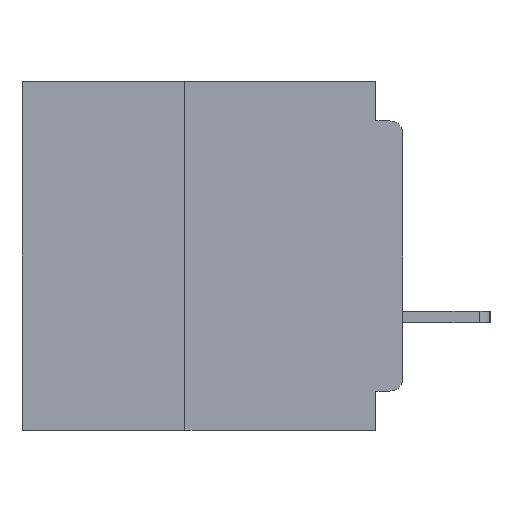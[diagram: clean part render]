
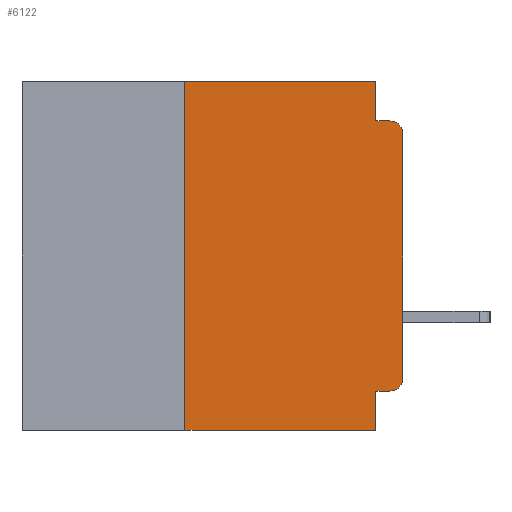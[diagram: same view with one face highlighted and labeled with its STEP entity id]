
A CAD part, left-side view. The second image highlights one B-rep face of the part: STEP entity #6122.
In plain terms, the highlighted planar face has unit normal (-1, 0, 0).
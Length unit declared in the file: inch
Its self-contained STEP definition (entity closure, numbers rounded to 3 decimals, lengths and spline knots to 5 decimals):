
#371 = ORIENTED_EDGE ( 'NONE', *, *, #23966, .T. ) ;
#382 = CARTESIAN_POINT ( 'NONE',  ( 0., 0.25, -0.4 ) ) ;
#475 = CIRCLE ( 'NONE', #38629, 0.015 ) ;
#1666 = VERTEX_POINT ( 'NONE', #8540 ) ;
#4003 = VERTEX_POINT ( 'NONE', #382 ) ;
#4031 = ORIENTED_EDGE ( 'NONE', *, *, #8198, .T. ) ;
#5573 = EDGE_CURVE ( 'NONE', #4003, #1666, #17565, .T. ) ;
#6122 = ADVANCED_FACE ( 'NONE', ( #43134 ), #41842, .F. ) ;
#7147 = CARTESIAN_POINT ( 'NONE',  ( 0., 0.015, -0.355 ) ) ;
#7319 = LINE ( 'NONE', #8482, #46742 ) ;
#7358 = VECTOR ( 'NONE', #42615, 39.37008 ) ;
#8198 = EDGE_CURVE ( 'NONE', #46707, #48323, #47639, .T. ) ;
#8482 = CARTESIAN_POINT ( 'NONE',  ( 0., 0.437, 0. ) ) ;
#8540 = CARTESIAN_POINT ( 'NONE',  ( 0., 0.031, -0.4 ) ) ;
#10639 = VECTOR ( 'NONE', #27097, 39.37008 ) ;
#11335 = LINE ( 'NONE', #21030, #31790 ) ;
#12871 = VERTEX_POINT ( 'NONE', #7147 ) ;
#12902 = AXIS2_PLACEMENT_3D ( 'NONE', #16876, #43560, #20738 ) ;
#13273 = CARTESIAN_POINT ( 'NONE',  ( 0., 0.437, -0.4 ) ) ;
#13705 = DIRECTION ( 'NONE',  ( 0., -1., 0. ) ) ;
#13744 = DIRECTION ( 'NONE',  ( 0., 0., 1. ) ) ;
#15393 = ORIENTED_EDGE ( 'NONE', *, *, #5573, .T. ) ;
#15849 = VERTEX_POINT ( 'NONE', #41831 ) ;
#16168 = EDGE_CURVE ( 'NONE', #4003, #17813, #24903, .T. ) ;
#16334 = DIRECTION ( 'NONE',  ( -1., 0., 0. ) ) ;
#16491 = CARTESIAN_POINT ( 'NONE',  ( 0., 0., -0.355 ) ) ;
#16876 = CARTESIAN_POINT ( 'NONE',  ( 0., 0.015, -0.06 ) ) ;
#16954 = EDGE_CURVE ( 'NONE', #17813, #47381, #7319, .T. ) ;
#17565 = LINE ( 'NONE', #13273, #18763 ) ;
#17813 = VERTEX_POINT ( 'NONE', #36691 ) ;
#17838 = ORIENTED_EDGE ( 'NONE', *, *, #25099, .F. ) ;
#18763 = VECTOR ( 'NONE', #13705, 39.37008 ) ;
#19045 = ORIENTED_EDGE ( 'NONE', *, *, #48656, .F. ) ;
#19424 = VECTOR ( 'NONE', #13744, 39.37008 ) ;
#19915 = LINE ( 'NONE', #16491, #27682 ) ;
#20049 = EDGE_LOOP ( 'NONE', ( #371, #4031, #19045, #44079, #21466, #37556, #15393, #22036, #17838, #45035 ) ) ;
#20738 = DIRECTION ( 'NONE',  ( 0., 0., -1. ) ) ;
#21030 = CARTESIAN_POINT ( 'NONE',  ( 0., 0., -0.045 ) ) ;
#21466 = ORIENTED_EDGE ( 'NONE', *, *, #16954, .F. ) ;
#22036 = ORIENTED_EDGE ( 'NONE', *, *, #36797, .F. ) ;
#22149 = LINE ( 'NONE', #38689, #10639 ) ;
#23005 = VERTEX_POINT ( 'NONE', #30158 ) ;
#23358 = CARTESIAN_POINT ( 'NONE',  ( 0., 0.031, -0.045 ) ) ;
#23966 = EDGE_CURVE ( 'NONE', #15849, #46707, #39679, .T. ) ;
#24005 = DIRECTION ( 'NONE',  ( 0., -1., 0. ) ) ;
#24903 = LINE ( 'NONE', #38187, #26095 ) ;
#25099 = EDGE_CURVE ( 'NONE', #12871, #23005, #19915, .T. ) ;
#25739 = CARTESIAN_POINT ( 'NONE',  ( 0., 0.015, -0.045 ) ) ;
#26095 = VECTOR ( 'NONE', #30747, 39.37008 ) ;
#26703 = EDGE_CURVE ( 'NONE', #47381, #49003, #22149, .T. ) ;
#26773 = EDGE_CURVE ( 'NONE', #12871, #15849, #475, .T. ) ;
#27097 = DIRECTION ( 'NONE',  ( 0., 0., -1. ) ) ;
#27682 = VECTOR ( 'NONE', #43173, 39.37008 ) ;
#30158 = CARTESIAN_POINT ( 'NONE',  ( 0., 0.031, -0.355 ) ) ;
#30747 = DIRECTION ( 'NONE',  ( 0., 0., 1. ) ) ;
#31790 = VECTOR ( 'NONE', #40145, 39.37008 ) ;
#36666 = CARTESIAN_POINT ( 'NONE',  ( 0., 0., 0. ) ) ;
#36691 = CARTESIAN_POINT ( 'NONE',  ( 0., 0.25, 0. ) ) ;
#36797 = EDGE_CURVE ( 'NONE', #23005, #1666, #49130, .T. ) ;
#37556 = ORIENTED_EDGE ( 'NONE', *, *, #16168, .F. ) ;
#38187 = CARTESIAN_POINT ( 'NONE',  ( 0., 0.25, -0.4 ) ) ;
#38629 = AXIS2_PLACEMENT_3D ( 'NONE', #39178, #16334, #43012 ) ;
#38689 = CARTESIAN_POINT ( 'NONE',  ( 0., 0.031, 0. ) ) ;
#38771 = CARTESIAN_POINT ( 'NONE',  ( 0., 0.031, -0.4 ) ) ;
#39178 = CARTESIAN_POINT ( 'NONE',  ( 0., 0.015, -0.34 ) ) ;
#39679 = LINE ( 'NONE', #36666, #19424 ) ;
#39924 = CARTESIAN_POINT ( 'NONE',  ( 0., 0., -0.06 ) ) ;
#40145 = DIRECTION ( 'NONE',  ( 0., -1., 0. ) ) ;
#41303 = DIRECTION ( 'NONE',  ( 0., 0., -1. ) ) ;
#41416 = DIRECTION ( 'NONE',  ( 1., 0., 0. ) ) ;
#41688 = CARTESIAN_POINT ( 'NONE',  ( 0., 0.437, 0. ) ) ;
#41831 = CARTESIAN_POINT ( 'NONE',  ( 0., 0., -0.34 ) ) ;
#41842 = PLANE ( 'NONE',  #48625 ) ;
#42615 = DIRECTION ( 'NONE',  ( 0., 0., -1. ) ) ;
#42915 = CARTESIAN_POINT ( 'NONE',  ( 0., 0.031, 0. ) ) ;
#43012 = DIRECTION ( 'NONE',  ( 0., 0., -1. ) ) ;
#43134 = FACE_OUTER_BOUND ( 'NONE', #20049, .T. ) ;
#43173 = DIRECTION ( 'NONE',  ( 0., 1., 0. ) ) ;
#43560 = DIRECTION ( 'NONE',  ( -1., 0., 0. ) ) ;
#44079 = ORIENTED_EDGE ( 'NONE', *, *, #26703, .F. ) ;
#45035 = ORIENTED_EDGE ( 'NONE', *, *, #26773, .T. ) ;
#46707 = VERTEX_POINT ( 'NONE', #39924 ) ;
#46742 = VECTOR ( 'NONE', #24005, 39.37008 ) ;
#47381 = VERTEX_POINT ( 'NONE', #42915 ) ;
#47639 = CIRCLE ( 'NONE', #12902, 0.015 ) ;
#48323 = VERTEX_POINT ( 'NONE', #25739 ) ;
#48625 = AXIS2_PLACEMENT_3D ( 'NONE', #41688, #41416, #41303 ) ;
#48656 = EDGE_CURVE ( 'NONE', #49003, #48323, #11335, .T. ) ;
#49003 = VERTEX_POINT ( 'NONE', #23358 ) ;
#49130 = LINE ( 'NONE', #38771, #7358 ) ;
